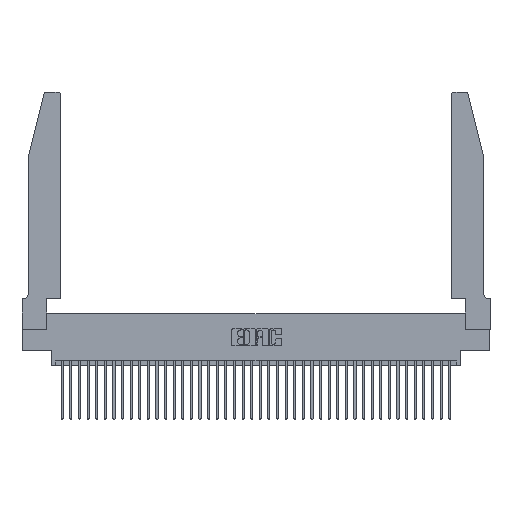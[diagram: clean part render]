
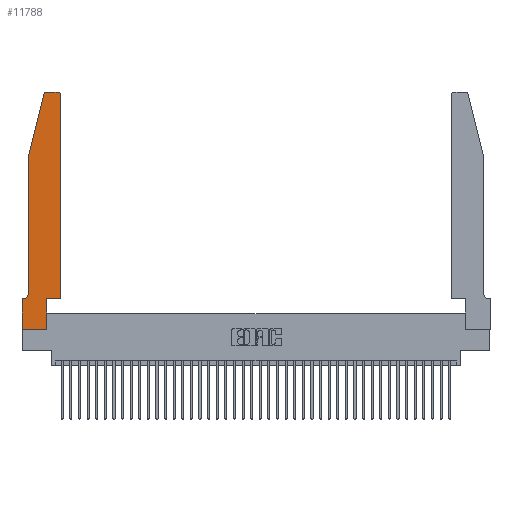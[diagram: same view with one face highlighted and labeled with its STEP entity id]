
A CAD part, top view. The second image highlights one B-rep face of the part: STEP entity #11788.
In plain terms, the highlighted planar face has unit normal (0, 0, 1).
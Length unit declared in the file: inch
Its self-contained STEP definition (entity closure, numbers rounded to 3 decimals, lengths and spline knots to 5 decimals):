
#213 = CARTESIAN_POINT ( 'NONE',  ( 0.4505, 0.35, 0.37 ) ) ;
#529 = EDGE_CURVE ( 'NONE', #29613, #1146, #25854, .T. ) ;
#757 = VECTOR ( 'NONE', #37679, 39.37008 ) ;
#888 = CARTESIAN_POINT ( 'NONE',  ( 0.2865, 0.35, 0.37 ) ) ;
#1102 = ORIENTED_EDGE ( 'NONE', *, *, #529, .T. ) ;
#1146 = VERTEX_POINT ( 'NONE', #10330 ) ;
#1290 = LINE ( 'NONE', #17922, #17178 ) ;
#2231 = AXIS2_PLACEMENT_3D ( 'NONE', #11908, #33555, #15024 ) ;
#2269 = CARTESIAN_POINT ( 'NONE',  ( 0.0755, 2., 0.37 ) ) ;
#2513 = ORIENTED_EDGE ( 'NONE', *, *, #6966, .T. ) ;
#2893 = CARTESIAN_POINT ( 'NONE',  ( 0.4205, 2.72, 0.37 ) ) ;
#3216 = ORIENTED_EDGE ( 'NONE', *, *, #40289, .T. ) ;
#3279 = VERTEX_POINT ( 'NONE', #28022 ) ;
#4098 = DIRECTION ( 'NONE',  ( 1., 0., 0. ) ) ;
#4405 = ORIENTED_EDGE ( 'NONE', *, *, #19029, .T. ) ;
#5531 = DIRECTION ( 'NONE',  ( -0.239, -0.971, 0. ) ) ;
#5888 = VERTEX_POINT ( 'NONE', #30762 ) ;
#5904 = ORIENTED_EDGE ( 'NONE', *, *, #29937, .T. ) ;
#5913 = AXIS2_PLACEMENT_3D ( 'NONE', #2893, #24842, #6153 ) ;
#6153 = DIRECTION ( 'NONE',  ( 1., 0., 0. ) ) ;
#6235 = ORIENTED_EDGE ( 'NONE', *, *, #31022, .T. ) ;
#6966 = EDGE_CURVE ( 'NONE', #5888, #32479, #13857, .T. ) ;
#7638 = EDGE_CURVE ( 'NONE', #31569, #10483, #37975, .T. ) ;
#8217 = VERTEX_POINT ( 'NONE', #15046 ) ;
#9000 = ORIENTED_EDGE ( 'NONE', *, *, #21082, .T. ) ;
#9068 = AXIS2_PLACEMENT_3D ( 'NONE', #19790, #22898, #4098 ) ;
#9524 = ORIENTED_EDGE ( 'NONE', *, *, #32077, .T. ) ;
#10330 = CARTESIAN_POINT ( 'NONE',  ( 0.4505, 2.72, 0.37 ) ) ;
#10420 = CARTESIAN_POINT ( 'NONE',  ( 0.0755, 2., 0.37 ) ) ;
#10483 = VERTEX_POINT ( 'NONE', #10420 ) ;
#10761 = VERTEX_POINT ( 'NONE', #11750 ) ;
#11351 = CIRCLE ( 'NONE', #2231, 0.07 ) ;
#11750 = CARTESIAN_POINT ( 'NONE',  ( 0.4205, 2.75, 0.37 ) ) ;
#11788 = ADVANCED_FACE ( 'NONE', ( #18440 ), #38265, .T. ) ;
#11908 = CARTESIAN_POINT ( 'NONE',  ( 0.0055, 0.42, 0.37 ) ) ;
#12233 = VECTOR ( 'NONE', #25410, 39.37008 ) ;
#12347 = VECTOR ( 'NONE', #5531, 39.37008 ) ;
#12894 = VECTOR ( 'NONE', #36177, 39.37008 ) ;
#13857 = LINE ( 'NONE', #33105, #12894 ) ;
#14562 = VECTOR ( 'NONE', #20817, 39.37008 ) ;
#15024 = DIRECTION ( 'NONE',  ( -1., 0., 0. ) ) ;
#15046 = CARTESIAN_POINT ( 'NONE',  ( 0., 0.35, 0.37 ) ) ;
#15072 = ORIENTED_EDGE ( 'NONE', *, *, #21175, .T. ) ;
#16805 = VECTOR ( 'NONE', #29989, 39.37008 ) ;
#16991 = CARTESIAN_POINT ( 'NONE',  ( 0.284, 2.72, 0.37 ) ) ;
#17178 = VECTOR ( 'NONE', #21034, 39.37008 ) ;
#17532 = CARTESIAN_POINT ( 'NONE',  ( 0.0755, 0.35, 0.37 ) ) ;
#17759 = LINE ( 'NONE', #17532, #16805 ) ;
#17922 = CARTESIAN_POINT ( 'NONE',  ( 0., 0., 0.37 ) ) ;
#18337 = ORIENTED_EDGE ( 'NONE', *, *, #38608, .T. ) ;
#18440 = FACE_OUTER_BOUND ( 'NONE', #26077, .T. ) ;
#18546 = DIRECTION ( 'NONE',  ( 0., -1., 0. ) ) ;
#19029 = EDGE_CURVE ( 'NONE', #3279, #8217, #17759, .T. ) ;
#19790 = CARTESIAN_POINT ( 'NONE',  ( 0., 0.35, 0.37 ) ) ;
#20108 = DIRECTION ( 'NONE',  ( 1., 0., 0. ) ) ;
#20498 = VERTEX_POINT ( 'NONE', #34147 ) ;
#20817 = DIRECTION ( 'NONE',  ( 1., 0., 0. ) ) ;
#21034 = DIRECTION ( 'NONE',  ( 0., -1., 0. ) ) ;
#21082 = EDGE_CURVE ( 'NONE', #21643, #3279, #11351, .T. ) ;
#21175 = EDGE_CURVE ( 'NONE', #10483, #21643, #31226, .T. ) ;
#21474 = VECTOR ( 'NONE', #25652, 39.37008 ) ;
#21643 = VERTEX_POINT ( 'NONE', #23784 ) ;
#22898 = DIRECTION ( 'NONE',  ( 0., 0., 1. ) ) ;
#23784 = CARTESIAN_POINT ( 'NONE',  ( 0.0755, 0.42, 0.37 ) ) ;
#24055 = CIRCLE ( 'NONE', #5913, 0.03 ) ;
#24842 = DIRECTION ( 'NONE',  ( 0., 0., 1. ) ) ;
#25044 = ORIENTED_EDGE ( 'NONE', *, *, #35485, .T. ) ;
#25074 = CIRCLE ( 'NONE', #28605, 0.03 ) ;
#25410 = DIRECTION ( 'NONE',  ( 1., 0., 0. ) ) ;
#25652 = DIRECTION ( 'NONE',  ( -1., 0., 0. ) ) ;
#25854 = LINE ( 'NONE', #213, #757 ) ;
#26077 = EDGE_LOOP ( 'NONE', ( #25044, #18337, #34730, #15072, #9000, #4405, #5904, #9524, #2513, #6235, #1102, #3216 ) ) ;
#26902 = CARTESIAN_POINT ( 'NONE',  ( 0., 0., 0.37 ) ) ;
#27887 = CARTESIAN_POINT ( 'NONE',  ( 0.0755, 2., 0.37 ) ) ;
#28022 = CARTESIAN_POINT ( 'NONE',  ( 0.0055, 0.35, 0.37 ) ) ;
#28544 = CARTESIAN_POINT ( 'NONE',  ( 0.4505, 0.35, 0.37 ) ) ;
#28605 = AXIS2_PLACEMENT_3D ( 'NONE', #16991, #38588, #20108 ) ;
#28705 = LINE ( 'NONE', #28544, #12233 ) ;
#29263 = VECTOR ( 'NONE', #18546, 39.37008 ) ;
#29613 = VERTEX_POINT ( 'NONE', #34841 ) ;
#29831 = VERTEX_POINT ( 'NONE', #32951 ) ;
#29937 = EDGE_CURVE ( 'NONE', #8217, #20498, #1290, .T. ) ;
#29989 = DIRECTION ( 'NONE',  ( -1., 0., 0. ) ) ;
#30762 = CARTESIAN_POINT ( 'NONE',  ( 0.2865, 0., 0.37 ) ) ;
#31022 = EDGE_CURVE ( 'NONE', #32479, #29613, #28705, .T. ) ;
#31063 = LINE ( 'NONE', #26902, #14562 ) ;
#31226 = LINE ( 'NONE', #27887, #29263 ) ;
#31569 = VERTEX_POINT ( 'NONE', #36897 ) ;
#32077 = EDGE_CURVE ( 'NONE', #20498, #5888, #31063, .T. ) ;
#32479 = VERTEX_POINT ( 'NONE', #888 ) ;
#32951 = CARTESIAN_POINT ( 'NONE',  ( 0.284, 2.75, 0.37 ) ) ;
#33105 = CARTESIAN_POINT ( 'NONE',  ( 0.2865, 0.35, 0.37 ) ) ;
#33555 = DIRECTION ( 'NONE',  ( 0., 0., -1. ) ) ;
#34147 = CARTESIAN_POINT ( 'NONE',  ( 0., 0., 0.37 ) ) ;
#34730 = ORIENTED_EDGE ( 'NONE', *, *, #7638, .T. ) ;
#34841 = CARTESIAN_POINT ( 'NONE',  ( 0.4505, 0.35, 0.37 ) ) ;
#35485 = EDGE_CURVE ( 'NONE', #10761, #29831, #38858, .T. ) ;
#36177 = DIRECTION ( 'NONE',  ( 0., 1., 0. ) ) ;
#36897 = CARTESIAN_POINT ( 'NONE',  ( 0.25487, 2.72718, 0.37 ) ) ;
#37679 = DIRECTION ( 'NONE',  ( 0., 1., 0. ) ) ;
#37930 = CARTESIAN_POINT ( 'NONE',  ( 0.2605, 2.75, 0.37 ) ) ;
#37975 = LINE ( 'NONE', #2269, #12347 ) ;
#38265 = PLANE ( 'NONE',  #9068 ) ;
#38588 = DIRECTION ( 'NONE',  ( 0., 0., 1. ) ) ;
#38608 = EDGE_CURVE ( 'NONE', #29831, #31569, #25074, .T. ) ;
#38858 = LINE ( 'NONE', #37930, #21474 ) ;
#40289 = EDGE_CURVE ( 'NONE', #1146, #10761, #24055, .T. ) ;
